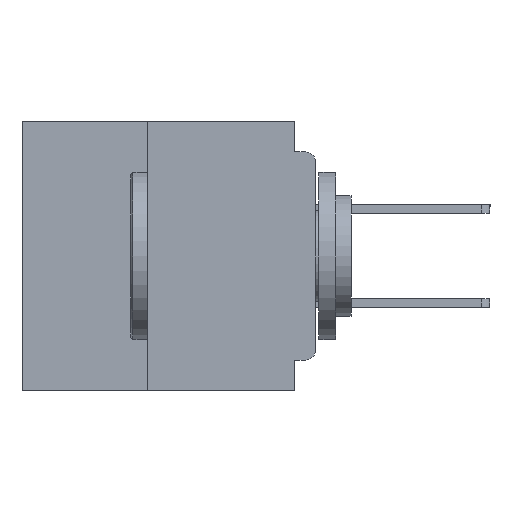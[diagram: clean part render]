
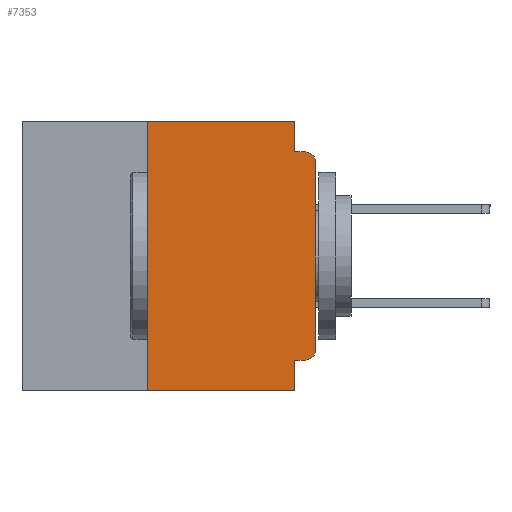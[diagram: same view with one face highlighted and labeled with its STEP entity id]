
A CAD part, left-side view. The second image highlights one B-rep face of the part: STEP entity #7353.
In plain terms, the highlighted planar face has unit normal (-1, 0, 0).
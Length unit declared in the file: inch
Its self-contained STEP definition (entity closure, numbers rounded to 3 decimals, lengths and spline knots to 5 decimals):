
#231 = VERTEX_POINT ( 'NONE', #58814 ) ;
#1641 = CARTESIAN_POINT ( 'NONE',  ( 0., 0.031, -0.4 ) ) ;
#2386 = LINE ( 'NONE', #49239, #54156 ) ;
#2566 = EDGE_CURVE ( 'NONE', #55361, #62466, #57561, .T. ) ;
#2579 = VERTEX_POINT ( 'NONE', #6523 ) ;
#2692 = ORIENTED_EDGE ( 'NONE', *, *, #62731, .T. ) ;
#3336 = EDGE_CURVE ( 'NONE', #16237, #48808, #23781, .T. ) ;
#5314 = AXIS2_PLACEMENT_3D ( 'NONE', #9362, #64434, #34462 ) ;
#6523 = CARTESIAN_POINT ( 'NONE',  ( 0., 0.031, -0.045 ) ) ;
#6810 = CARTESIAN_POINT ( 'NONE',  ( 0., 0., -0.06 ) ) ;
#7353 = ADVANCED_FACE ( 'NONE', ( #23920 ), #19439, .F. ) ;
#8421 = LINE ( 'NONE', #1641, #61627 ) ;
#8509 = LINE ( 'NONE', #10341, #60187 ) ;
#8680 = DIRECTION ( 'NONE',  ( 0., 0., -1. ) ) ;
#9030 = DIRECTION ( 'NONE',  ( -1., 0., 0. ) ) ;
#9255 = ORIENTED_EDGE ( 'NONE', *, *, #2566, .T. ) ;
#9362 = CARTESIAN_POINT ( 'NONE',  ( 0., 0.437, 0. ) ) ;
#9386 = CARTESIAN_POINT ( 'NONE',  ( 0., 0.015, -0.34 ) ) ;
#9913 = ORIENTED_EDGE ( 'NONE', *, *, #37320, .F. ) ;
#10341 = CARTESIAN_POINT ( 'NONE',  ( 0., 0.437, 0. ) ) ;
#10774 = DIRECTION ( 'NONE',  ( 0., 0., 1. ) ) ;
#11196 = ORIENTED_EDGE ( 'NONE', *, *, #3336, .T. ) ;
#11682 = VECTOR ( 'NONE', #45424, 39.37008 ) ;
#12301 = VECTOR ( 'NONE', #10774, 39.37008 ) ;
#13899 = LINE ( 'NONE', #50860, #12301 ) ;
#14223 = DIRECTION ( 'NONE',  ( 0., 1., 0. ) ) ;
#15226 = CARTESIAN_POINT ( 'NONE',  ( 0., 0.015, -0.045 ) ) ;
#15438 = CARTESIAN_POINT ( 'NONE',  ( 0., 0.437, -0.4 ) ) ;
#16038 = EDGE_CURVE ( 'NONE', #18159, #56549, #8509, .T. ) ;
#16056 = DIRECTION ( 'NONE',  ( 0., 0., -1. ) ) ;
#16130 = DIRECTION ( 'NONE',  ( -1., 0., 0. ) ) ;
#16175 = CARTESIAN_POINT ( 'NONE',  ( 0., 0.015, -0.06 ) ) ;
#16237 = VERTEX_POINT ( 'NONE', #6810 ) ;
#17422 = VECTOR ( 'NONE', #41317, 39.37008 ) ;
#18070 = ORIENTED_EDGE ( 'NONE', *, *, #57134, .T. ) ;
#18159 = VERTEX_POINT ( 'NONE', #63724 ) ;
#19439 = PLANE ( 'NONE',  #5314 ) ;
#19872 = EDGE_LOOP ( 'NONE', ( #18070, #11196, #20358, #29190, #51836, #59296, #2692, #9913, #38862, #9255 ) ) ;
#20358 = ORIENTED_EDGE ( 'NONE', *, *, #34813, .F. ) ;
#21041 = AXIS2_PLACEMENT_3D ( 'NONE', #9386, #9030, #8680 ) ;
#22294 = CARTESIAN_POINT ( 'NONE',  ( 0., 0.031, -0.355 ) ) ;
#23407 = CARTESIAN_POINT ( 'NONE',  ( 0., 0., 0. ) ) ;
#23701 = CARTESIAN_POINT ( 'NONE',  ( 0., 0.031, 0. ) ) ;
#23781 = CIRCLE ( 'NONE', #55458, 0.015 ) ;
#23920 = FACE_OUTER_BOUND ( 'NONE', #19872, .T. ) ;
#26341 = EDGE_CURVE ( 'NONE', #56549, #2579, #48837, .T. ) ;
#28392 = DIRECTION ( 'NONE',  ( 0., 0., 1. ) ) ;
#29190 = ORIENTED_EDGE ( 'NONE', *, *, #26341, .F. ) ;
#32418 = CARTESIAN_POINT ( 'NONE',  ( 0., 0., -0.34 ) ) ;
#34462 = DIRECTION ( 'NONE',  ( 0., 0., -1. ) ) ;
#34813 = EDGE_CURVE ( 'NONE', #2579, #48808, #44046, .T. ) ;
#36590 = DIRECTION ( 'NONE',  ( 0., 0., -1. ) ) ;
#37156 = CARTESIAN_POINT ( 'NONE',  ( 0., 0.031, 0. ) ) ;
#37320 = EDGE_CURVE ( 'NONE', #60301, #231, #8421, .T. ) ;
#38264 = LINE ( 'NONE', #15438, #11682 ) ;
#38862 = ORIENTED_EDGE ( 'NONE', *, *, #55419, .F. ) ;
#41317 = DIRECTION ( 'NONE',  ( 0., -1., 0. ) ) ;
#42111 = VECTOR ( 'NONE', #28392, 39.37008 ) ;
#43974 = CARTESIAN_POINT ( 'NONE',  ( 0., 0.015, -0.355 ) ) ;
#44046 = LINE ( 'NONE', #61206, #17422 ) ;
#45290 = LINE ( 'NONE', #23407, #42111 ) ;
#45424 = DIRECTION ( 'NONE',  ( 0., -1., 0. ) ) ;
#45857 = EDGE_CURVE ( 'NONE', #55856, #18159, #13899, .T. ) ;
#47260 = VECTOR ( 'NONE', #62134, 39.37008 ) ;
#48808 = VERTEX_POINT ( 'NONE', #15226 ) ;
#48837 = LINE ( 'NONE', #37156, #47260 ) ;
#49239 = CARTESIAN_POINT ( 'NONE',  ( 0., 0., -0.355 ) ) ;
#50860 = CARTESIAN_POINT ( 'NONE',  ( 0., 0.25, -0.4 ) ) ;
#51836 = ORIENTED_EDGE ( 'NONE', *, *, #16038, .F. ) ;
#54156 = VECTOR ( 'NONE', #14223, 39.37008 ) ;
#55361 = VERTEX_POINT ( 'NONE', #43974 ) ;
#55419 = EDGE_CURVE ( 'NONE', #55361, #60301, #2386, .T. ) ;
#55458 = AXIS2_PLACEMENT_3D ( 'NONE', #16175, #16130, #16056 ) ;
#55856 = VERTEX_POINT ( 'NONE', #62651 ) ;
#56549 = VERTEX_POINT ( 'NONE', #23701 ) ;
#57134 = EDGE_CURVE ( 'NONE', #62466, #16237, #45290, .T. ) ;
#57561 = CIRCLE ( 'NONE', #21041, 0.015 ) ;
#58814 = CARTESIAN_POINT ( 'NONE',  ( 0., 0.031, -0.4 ) ) ;
#59296 = ORIENTED_EDGE ( 'NONE', *, *, #45857, .F. ) ;
#60187 = VECTOR ( 'NONE', #60444, 39.37008 ) ;
#60301 = VERTEX_POINT ( 'NONE', #22294 ) ;
#60444 = DIRECTION ( 'NONE',  ( 0., -1., 0. ) ) ;
#61206 = CARTESIAN_POINT ( 'NONE',  ( 0., 0., -0.045 ) ) ;
#61627 = VECTOR ( 'NONE', #36590, 39.37008 ) ;
#62134 = DIRECTION ( 'NONE',  ( 0., 0., -1. ) ) ;
#62466 = VERTEX_POINT ( 'NONE', #32418 ) ;
#62651 = CARTESIAN_POINT ( 'NONE',  ( 0., 0.25, -0.4 ) ) ;
#62731 = EDGE_CURVE ( 'NONE', #55856, #231, #38264, .T. ) ;
#63724 = CARTESIAN_POINT ( 'NONE',  ( 0., 0.25, 0. ) ) ;
#64434 = DIRECTION ( 'NONE',  ( 1., 0., 0. ) ) ;
